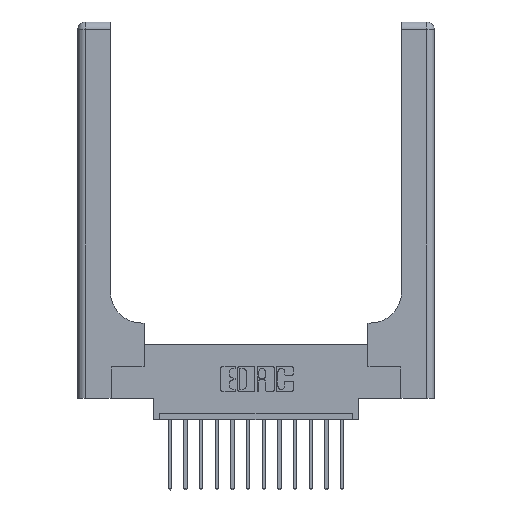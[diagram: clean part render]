
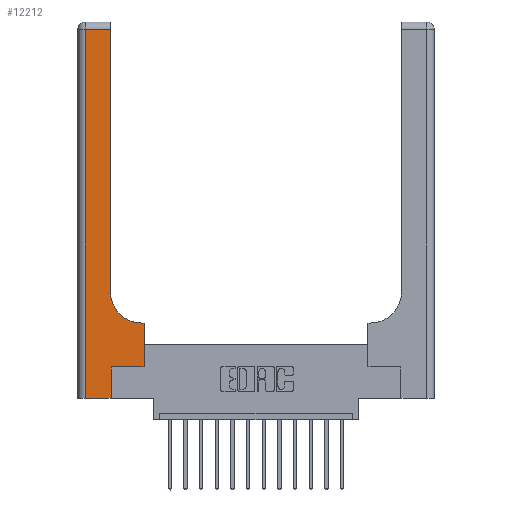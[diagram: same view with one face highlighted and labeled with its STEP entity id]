
A CAD part, top view. The second image highlights one B-rep face of the part: STEP entity #12212.
In plain terms, the highlighted planar face has unit normal (0, 0, 1).
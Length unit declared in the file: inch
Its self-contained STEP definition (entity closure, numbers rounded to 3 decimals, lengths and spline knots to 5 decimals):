
#45 = CARTESIAN_POINT ( 'NONE',  ( 0.265, 0.25, 0.37 ) ) ;
#96 = ORIENTED_EDGE ( 'NONE', *, *, #12190, .T. ) ;
#581 = DIRECTION ( 'NONE',  ( 1., 0., 0. ) ) ;
#687 = CARTESIAN_POINT ( 'NONE',  ( 0.265, 0., 0.37 ) ) ;
#1448 = CARTESIAN_POINT ( 'NONE',  ( 0.265, 0.25, 0.37 ) ) ;
#1486 = CARTESIAN_POINT ( 'NONE',  ( 0.26, 3., 0.37 ) ) ;
#1505 = CARTESIAN_POINT ( 'NONE',  ( 0.26, 0.6, 0.37 ) ) ;
#1985 = AXIS2_PLACEMENT_3D ( 'NONE', #13896, #13772, #3422 ) ;
#2162 = LINE ( 'NONE', #1448, #10426 ) ;
#2213 = ORIENTED_EDGE ( 'NONE', *, *, #11052, .T. ) ;
#2254 = VECTOR ( 'NONE', #13610, 39.37008 ) ;
#2894 = VECTOR ( 'NONE', #6618, 39.37008 ) ;
#3422 = DIRECTION ( 'NONE',  ( -1., 0., 0. ) ) ;
#3529 = VECTOR ( 'NONE', #8243, 39.37008 ) ;
#3777 = LINE ( 'NONE', #1505, #16361 ) ;
#4151 = CARTESIAN_POINT ( 'NONE',  ( 0.06, 2.94, 0.37 ) ) ;
#4152 = ORIENTED_EDGE ( 'NONE', *, *, #7510, .T. ) ;
#4409 = CARTESIAN_POINT ( 'NONE',  ( 0.51, 0.6, 0.37 ) ) ;
#4632 = VERTEX_POINT ( 'NONE', #45 ) ;
#4667 = DIRECTION ( 'NONE',  ( 1., 0., 0. ) ) ;
#4677 = LINE ( 'NONE', #15546, #6881 ) ;
#5088 = CARTESIAN_POINT ( 'NONE',  ( 0.26, 2.94, 0.37 ) ) ;
#5246 = LINE ( 'NONE', #6841, #11731 ) ;
#5552 = ORIENTED_EDGE ( 'NONE', *, *, #8600, .T. ) ;
#5573 = LINE ( 'NONE', #13945, #14521 ) ;
#5818 = VERTEX_POINT ( 'NONE', #12771 ) ;
#6267 = CARTESIAN_POINT ( 'NONE',  ( 0.528, 0.6, 0.37 ) ) ;
#6618 = DIRECTION ( 'NONE',  ( 0., 1., 0. ) ) ;
#6716 = EDGE_CURVE ( 'NONE', #7646, #4632, #15227, .T. ) ;
#6841 = CARTESIAN_POINT ( 'NONE',  ( 0.06, 3., 0.37 ) ) ;
#6881 = VECTOR ( 'NONE', #9177, 39.37008 ) ;
#7201 = VERTEX_POINT ( 'NONE', #4409 ) ;
#7510 = EDGE_CURVE ( 'NONE', #14004, #5818, #5246, .T. ) ;
#7646 = VERTEX_POINT ( 'NONE', #687 ) ;
#8243 = DIRECTION ( 'NONE',  ( 0., 1., 0. ) ) ;
#8379 = CARTESIAN_POINT ( 'NONE',  ( 0.51, 0.85, 0.37 ) ) ;
#8600 = EDGE_CURVE ( 'NONE', #16229, #14004, #4677, .T. ) ;
#9177 = DIRECTION ( 'NONE',  ( -1., 0., 0. ) ) ;
#9325 = VERTEX_POINT ( 'NONE', #10684 ) ;
#9331 = DIRECTION ( 'NONE',  ( 1., 0., 0. ) ) ;
#9681 = DIRECTION ( 'NONE',  ( 0., 0., -1. ) ) ;
#9786 = CARTESIAN_POINT ( 'NONE',  ( 0.265, 0., 0.37 ) ) ;
#10314 = VERTEX_POINT ( 'NONE', #10621 ) ;
#10426 = VECTOR ( 'NONE', #9331, 39.37008 ) ;
#10523 = DIRECTION ( 'NONE',  ( -1., 0., 0. ) ) ;
#10621 = CARTESIAN_POINT ( 'NONE',  ( 0.528, 0.25, 0.37 ) ) ;
#10684 = CARTESIAN_POINT ( 'NONE',  ( 0.26, 0.85, 0.37 ) ) ;
#11052 = EDGE_CURVE ( 'NONE', #4632, #10314, #2162, .T. ) ;
#11152 = EDGE_CURVE ( 'NONE', #16069, #7201, #3777, .T. ) ;
#11153 = PLANE ( 'NONE',  #1985 ) ;
#11341 = EDGE_CURVE ( 'NONE', #7201, #9325, #11855, .T. ) ;
#11731 = VECTOR ( 'NONE', #14687, 39.37008 ) ;
#11855 = CIRCLE ( 'NONE', #15671, 0.25 ) ;
#12190 = EDGE_CURVE ( 'NONE', #5818, #7646, #5573, .T. ) ;
#12212 = ADVANCED_FACE ( 'NONE', ( #12282 ), #11153, .F. ) ;
#12241 = ORIENTED_EDGE ( 'NONE', *, *, #11341, .T. ) ;
#12282 = FACE_OUTER_BOUND ( 'NONE', #13152, .T. ) ;
#12771 = CARTESIAN_POINT ( 'NONE',  ( 0.06, 0., 0.37 ) ) ;
#12973 = ORIENTED_EDGE ( 'NONE', *, *, #13929, .T. ) ;
#13142 = EDGE_CURVE ( 'NONE', #10314, #16069, #16315, .T. ) ;
#13152 = EDGE_LOOP ( 'NONE', ( #12973, #5552, #4152, #96, #15691, #2213, #16763, #16522, #12241 ) ) ;
#13358 = CARTESIAN_POINT ( 'NONE',  ( 0.528, 0.25, 0.37 ) ) ;
#13610 = DIRECTION ( 'NONE',  ( 0., 1., 0. ) ) ;
#13772 = DIRECTION ( 'NONE',  ( 0., 0., -1. ) ) ;
#13896 = CARTESIAN_POINT ( 'NONE',  ( 0., 3., 0.37 ) ) ;
#13929 = EDGE_CURVE ( 'NONE', #9325, #16229, #15268, .T. ) ;
#13945 = CARTESIAN_POINT ( 'NONE',  ( 0., 0., 0.37 ) ) ;
#14004 = VERTEX_POINT ( 'NONE', #4151 ) ;
#14521 = VECTOR ( 'NONE', #4667, 39.37008 ) ;
#14687 = DIRECTION ( 'NONE',  ( 0., -1., 0. ) ) ;
#15227 = LINE ( 'NONE', #9786, #2254 ) ;
#15268 = LINE ( 'NONE', #1486, #2894 ) ;
#15546 = CARTESIAN_POINT ( 'NONE',  ( 0., 2.94, 0.37 ) ) ;
#15671 = AXIS2_PLACEMENT_3D ( 'NONE', #8379, #9681, #581 ) ;
#15691 = ORIENTED_EDGE ( 'NONE', *, *, #6716, .T. ) ;
#16069 = VERTEX_POINT ( 'NONE', #6267 ) ;
#16229 = VERTEX_POINT ( 'NONE', #5088 ) ;
#16315 = LINE ( 'NONE', #13358, #3529 ) ;
#16361 = VECTOR ( 'NONE', #10523, 39.37008 ) ;
#16522 = ORIENTED_EDGE ( 'NONE', *, *, #11152, .T. ) ;
#16763 = ORIENTED_EDGE ( 'NONE', *, *, #13142, .T. ) ;
